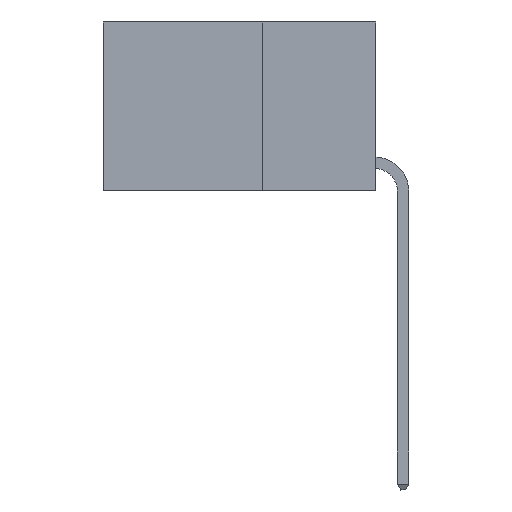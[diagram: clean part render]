
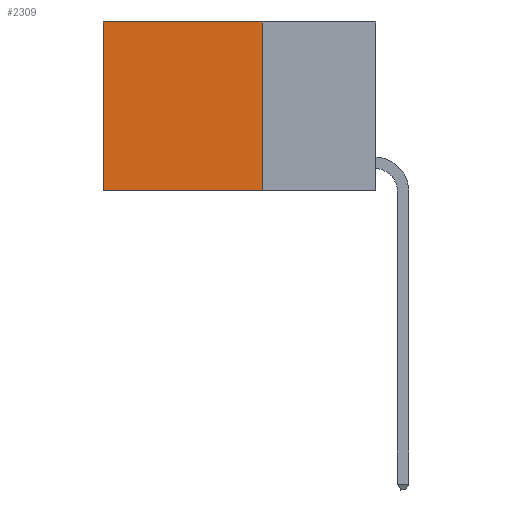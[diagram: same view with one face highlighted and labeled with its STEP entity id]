
A CAD part, left-side view. The second image highlights one B-rep face of the part: STEP entity #2309.
In plain terms, the highlighted planar face has unit normal (-1, 0, 0).
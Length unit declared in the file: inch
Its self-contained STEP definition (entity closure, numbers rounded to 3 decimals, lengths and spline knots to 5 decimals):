
#27 = LINE ( 'NONE', #1687, #1401 ) ;
#608 = EDGE_LOOP ( 'NONE', ( #11747, #9176, #7183, #5102 ) ) ;
#1101 = EDGE_CURVE ( 'NONE', #1352, #5046, #12035, .T. ) ;
#1152 = VERTEX_POINT ( 'NONE', #8809 ) ;
#1352 = VERTEX_POINT ( 'NONE', #5467 ) ;
#1401 = VECTOR ( 'NONE', #2096, 39.37008 ) ;
#1441 = FACE_OUTER_BOUND ( 'NONE', #608, .T. ) ;
#1687 = CARTESIAN_POINT ( 'NONE',  ( 0.2625, 0.25, 0. ) ) ;
#2096 = DIRECTION ( 'NONE',  ( 0., 1., 0. ) ) ;
#2309 = ADVANCED_FACE ( 'NONE', ( #1441 ), #3445, .F. ) ;
#3384 = DIRECTION ( 'NONE',  ( 0., 0., -1. ) ) ;
#3432 = DIRECTION ( 'NONE',  ( 1., 0., 0. ) ) ;
#3445 = PLANE ( 'NONE',  #10093 ) ;
#3623 = CARTESIAN_POINT ( 'NONE',  ( 0.2625, 0.25, 0. ) ) ;
#4289 = VERTEX_POINT ( 'NONE', #9002 ) ;
#4603 = CARTESIAN_POINT ( 'NONE',  ( 0.2625, 0.6, -0.37 ) ) ;
#5046 = VERTEX_POINT ( 'NONE', #4603 ) ;
#5102 = ORIENTED_EDGE ( 'NONE', *, *, #5464, .T. ) ;
#5160 = VECTOR ( 'NONE', #5871, 39.37008 ) ;
#5280 = VECTOR ( 'NONE', #5468, 39.37008 ) ;
#5464 = EDGE_CURVE ( 'NONE', #4289, #1152, #27, .T. ) ;
#5467 = CARTESIAN_POINT ( 'NONE',  ( 0.2625, 0.25, -0.37 ) ) ;
#5468 = DIRECTION ( 'NONE',  ( 0., 0., -1. ) ) ;
#5796 = CARTESIAN_POINT ( 'NONE',  ( 0.2625, 0.25, -0.37 ) ) ;
#5871 = DIRECTION ( 'NONE',  ( 0., 1., 0. ) ) ;
#7082 = DIRECTION ( 'NONE',  ( 0., 0., -1. ) ) ;
#7183 = ORIENTED_EDGE ( 'NONE', *, *, #12169, .F. ) ;
#8809 = CARTESIAN_POINT ( 'NONE',  ( 0.2625, 0.6, 0. ) ) ;
#9002 = CARTESIAN_POINT ( 'NONE',  ( 0.2625, 0.25, 0. ) ) ;
#9176 = ORIENTED_EDGE ( 'NONE', *, *, #1101, .F. ) ;
#9471 = CARTESIAN_POINT ( 'NONE',  ( 0.2625, 0.25, 0. ) ) ;
#9782 = VECTOR ( 'NONE', #7082, 39.37008 ) ;
#10093 = AXIS2_PLACEMENT_3D ( 'NONE', #3623, #3432, #3384 ) ;
#10251 = EDGE_CURVE ( 'NONE', #1152, #5046, #12285, .T. ) ;
#11045 = CARTESIAN_POINT ( 'NONE',  ( 0.2625, 0.6, 0. ) ) ;
#11747 = ORIENTED_EDGE ( 'NONE', *, *, #10251, .T. ) ;
#12035 = LINE ( 'NONE', #5796, #5160 ) ;
#12169 = EDGE_CURVE ( 'NONE', #4289, #1352, #13082, .T. ) ;
#12285 = LINE ( 'NONE', #11045, #9782 ) ;
#13082 = LINE ( 'NONE', #9471, #5280 ) ;
